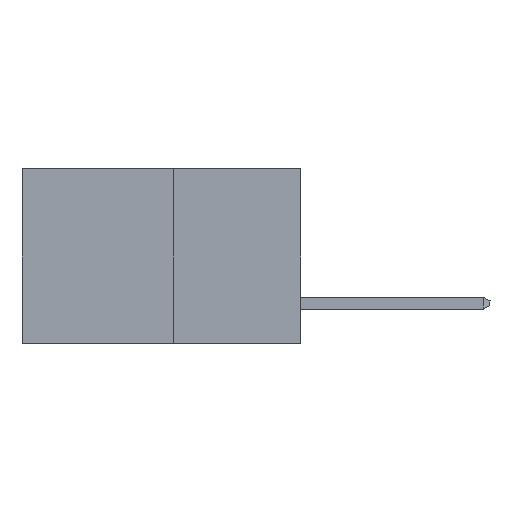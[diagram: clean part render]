
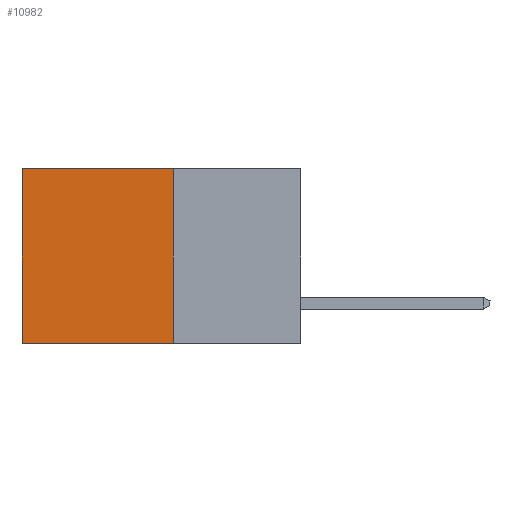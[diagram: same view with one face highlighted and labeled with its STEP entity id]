
A CAD part, left-side view. The second image highlights one B-rep face of the part: STEP entity #10982.
In plain terms, the highlighted planar face has unit normal (-1, 0, 0).
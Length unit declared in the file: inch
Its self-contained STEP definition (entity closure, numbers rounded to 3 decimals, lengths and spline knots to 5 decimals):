
#48 = DIRECTION ( 'NONE',  ( 0., 0., -1. ) ) ;
#517 = CARTESIAN_POINT ( 'NONE',  ( 0.277, 0.27, -0.37 ) ) ;
#826 = EDGE_CURVE ( 'NONE', #2599, #7225, #4541, .T. ) ;
#1169 = CARTESIAN_POINT ( 'NONE',  ( 0.277, 0.27, 0. ) ) ;
#1513 = EDGE_CURVE ( 'NONE', #8917, #7225, #2636, .T. ) ;
#2275 = CARTESIAN_POINT ( 'NONE',  ( 0.277, 0.27, -0.37 ) ) ;
#2285 = ORIENTED_EDGE ( 'NONE', *, *, #826, .T. ) ;
#2301 = ORIENTED_EDGE ( 'NONE', *, *, #1513, .F. ) ;
#2397 = EDGE_CURVE ( 'NONE', #8294, #2599, #7188, .T. ) ;
#2398 = DIRECTION ( 'NONE',  ( 0., 0., -1. ) ) ;
#2489 = EDGE_CURVE ( 'NONE', #8294, #8917, #3944, .T. ) ;
#2599 = VERTEX_POINT ( 'NONE', #9104 ) ;
#2636 = LINE ( 'NONE', #6808, #12186 ) ;
#3944 = LINE ( 'NONE', #2275, #6261 ) ;
#4416 = DIRECTION ( 'NONE',  ( 0., 1., 0. ) ) ;
#4541 = LINE ( 'NONE', #8209, #11797 ) ;
#5093 = EDGE_LOOP ( 'NONE', ( #2285, #2301, #7983, #7408 ) ) ;
#5668 = CARTESIAN_POINT ( 'NONE',  ( 0.277, 0.27, 0. ) ) ;
#6209 = DIRECTION ( 'NONE',  ( 1., 0., 0. ) ) ;
#6261 = VECTOR ( 'NONE', #2398, 39.37008 ) ;
#6406 = AXIS2_PLACEMENT_3D ( 'NONE', #11835, #6209, #48 ) ;
#6808 = CARTESIAN_POINT ( 'NONE',  ( 0.277, 0.27, -0.37 ) ) ;
#7156 = PLANE ( 'NONE',  #6406 ) ;
#7188 = LINE ( 'NONE', #5668, #12660 ) ;
#7225 = VERTEX_POINT ( 'NONE', #10928 ) ;
#7408 = ORIENTED_EDGE ( 'NONE', *, *, #2397, .T. ) ;
#7983 = ORIENTED_EDGE ( 'NONE', *, *, #2489, .F. ) ;
#8050 = DIRECTION ( 'NONE',  ( 0., 1., 0. ) ) ;
#8209 = CARTESIAN_POINT ( 'NONE',  ( 0.277, 0.59, -0.37 ) ) ;
#8294 = VERTEX_POINT ( 'NONE', #1169 ) ;
#8917 = VERTEX_POINT ( 'NONE', #517 ) ;
#9104 = CARTESIAN_POINT ( 'NONE',  ( 0.277, 0.59, 0. ) ) ;
#10139 = FACE_OUTER_BOUND ( 'NONE', #5093, .T. ) ;
#10928 = CARTESIAN_POINT ( 'NONE',  ( 0.277, 0.59, -0.37 ) ) ;
#10982 = ADVANCED_FACE ( 'NONE', ( #10139 ), #7156, .F. ) ;
#10985 = DIRECTION ( 'NONE',  ( 0., 0., -1. ) ) ;
#11797 = VECTOR ( 'NONE', #10985, 39.37008 ) ;
#11835 = CARTESIAN_POINT ( 'NONE',  ( 0.277, 0.27, -0.37 ) ) ;
#12186 = VECTOR ( 'NONE', #8050, 39.37008 ) ;
#12660 = VECTOR ( 'NONE', #4416, 39.37008 ) ;
